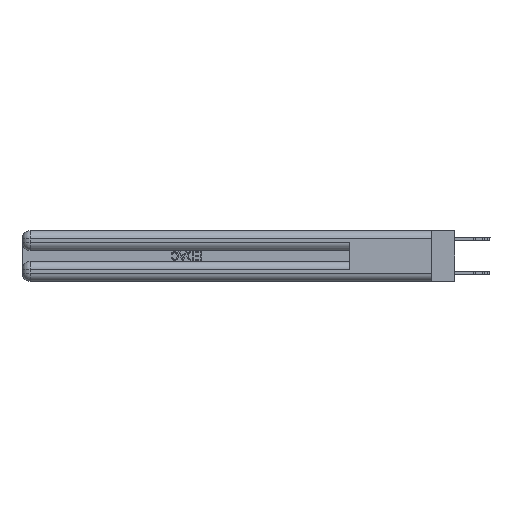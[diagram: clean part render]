
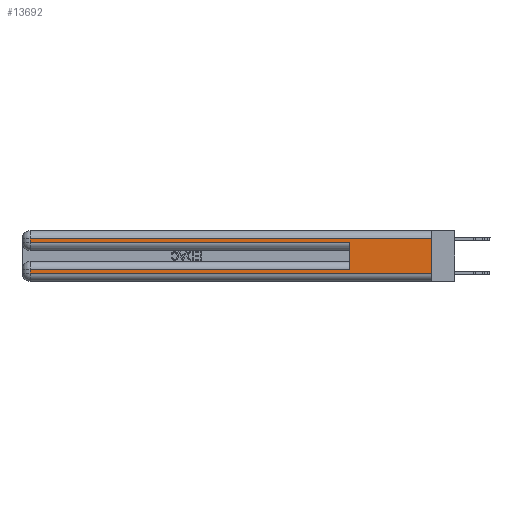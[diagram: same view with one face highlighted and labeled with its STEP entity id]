
A CAD part, left-side view. The second image highlights one B-rep face of the part: STEP entity #13692.
In plain terms, the highlighted planar face has unit normal (-1, 0, 0).
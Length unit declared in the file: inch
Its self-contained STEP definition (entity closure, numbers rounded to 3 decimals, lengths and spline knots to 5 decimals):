
#236 = LINE ( 'NONE', #10302, #12763 ) ;
#909 = EDGE_CURVE ( 'NONE', #18270, #22150, #18606, .T. ) ;
#1221 = CARTESIAN_POINT ( 'NONE',  ( 0., 2.94, 0.37 ) ) ;
#1953 = VECTOR ( 'NONE', #5404, 39.37008 ) ;
#2802 = EDGE_CURVE ( 'NONE', #17576, #24752, #4021, .T. ) ;
#3401 = LINE ( 'NONE', #13656, #1953 ) ;
#4021 = LINE ( 'NONE', #1221, #25824 ) ;
#4067 = VERTEX_POINT ( 'NONE', #9321 ) ;
#4225 = EDGE_CURVE ( 'NONE', #4067, #22150, #236, .T. ) ;
#4426 = CARTESIAN_POINT ( 'NONE',  ( 0., 2.94, 0.085 ) ) ;
#4803 = VECTOR ( 'NONE', #28341, 39.37008 ) ;
#4826 = DIRECTION ( 'NONE',  ( 0., 1., 0. ) ) ;
#5348 = CARTESIAN_POINT ( 'NONE',  ( 0., 0.6, 0.085 ) ) ;
#5404 = DIRECTION ( 'NONE',  ( 0., 0., -1. ) ) ;
#5659 = VECTOR ( 'NONE', #22503, 39.37008 ) ;
#7192 = ORIENTED_EDGE ( 'NONE', *, *, #2802, .T. ) ;
#8212 = CARTESIAN_POINT ( 'NONE',  ( 0., 0., 0.06 ) ) ;
#8763 = VECTOR ( 'NONE', #24407, 39.37008 ) ;
#9306 = DIRECTION ( 'NONE',  ( 1., 0., 0. ) ) ;
#9321 = CARTESIAN_POINT ( 'NONE',  ( 0., 0., 0.31 ) ) ;
#9666 = VERTEX_POINT ( 'NONE', #4426 ) ;
#9867 = CARTESIAN_POINT ( 'NONE',  ( 0., 2.94, 0.31 ) ) ;
#10302 = CARTESIAN_POINT ( 'NONE',  ( 0., 0., 0.37 ) ) ;
#10973 = ORIENTED_EDGE ( 'NONE', *, *, #909, .T. ) ;
#11294 = DIRECTION ( 'NONE',  ( 0., 0., -1. ) ) ;
#11939 = CARTESIAN_POINT ( 'NONE',  ( 0., 0., 0.085 ) ) ;
#12763 = VECTOR ( 'NONE', #25305, 39.37008 ) ;
#12928 = DIRECTION ( 'NONE',  ( 0., 0., 1. ) ) ;
#13603 = DIRECTION ( 'NONE',  ( 0., 0., -1. ) ) ;
#13656 = CARTESIAN_POINT ( 'NONE',  ( 0., 2.94, 0.37 ) ) ;
#13684 = VECTOR ( 'NONE', #12928, 39.37008 ) ;
#13692 = ADVANCED_FACE ( 'NONE', ( #31259 ), #19378, .F. ) ;
#14839 = CARTESIAN_POINT ( 'NONE',  ( 0., 0., 0.285 ) ) ;
#15610 = ORIENTED_EDGE ( 'NONE', *, *, #18496, .T. ) ;
#16903 = LINE ( 'NONE', #24815, #5659 ) ;
#17576 = VERTEX_POINT ( 'NONE', #9867 ) ;
#18212 = VERTEX_POINT ( 'NONE', #5348 ) ;
#18270 = VERTEX_POINT ( 'NONE', #20526 ) ;
#18496 = EDGE_CURVE ( 'NONE', #18212, #9666, #29753, .T. ) ;
#18606 = LINE ( 'NONE', #8212, #4803 ) ;
#19378 = PLANE ( 'NONE',  #30938 ) ;
#20526 = CARTESIAN_POINT ( 'NONE',  ( 0., 2.94, 0.06 ) ) ;
#20727 = EDGE_CURVE ( 'NONE', #24752, #26702, #29842, .T. ) ;
#21183 = CARTESIAN_POINT ( 'NONE',  ( 0., 0., 0.37 ) ) ;
#21469 = CARTESIAN_POINT ( 'NONE',  ( 0., 0.6, 0.285 ) ) ;
#21498 = EDGE_CURVE ( 'NONE', #9666, #18270, #3401, .T. ) ;
#21579 = ORIENTED_EDGE ( 'NONE', *, *, #22158, .T. ) ;
#21739 = CARTESIAN_POINT ( 'NONE',  ( 0., 2.94, 0.285 ) ) ;
#22150 = VERTEX_POINT ( 'NONE', #25139 ) ;
#22158 = EDGE_CURVE ( 'NONE', #4067, #17576, #16903, .T. ) ;
#22503 = DIRECTION ( 'NONE',  ( 0., 1., 0. ) ) ;
#23049 = ORIENTED_EDGE ( 'NONE', *, *, #26531, .F. ) ;
#23849 = ORIENTED_EDGE ( 'NONE', *, *, #20727, .T. ) ;
#24407 = DIRECTION ( 'NONE',  ( 0., -1., 0. ) ) ;
#24712 = EDGE_LOOP ( 'NONE', ( #29784, #21579, #7192, #23849, #23049, #15610, #28738, #10973 ) ) ;
#24752 = VERTEX_POINT ( 'NONE', #21739 ) ;
#24815 = CARTESIAN_POINT ( 'NONE',  ( 0., 0., 0.31 ) ) ;
#25130 = LINE ( 'NONE', #25606, #13684 ) ;
#25139 = CARTESIAN_POINT ( 'NONE',  ( 0., 0., 0.06 ) ) ;
#25305 = DIRECTION ( 'NONE',  ( 0., 0., -1. ) ) ;
#25606 = CARTESIAN_POINT ( 'NONE',  ( 0., 0.6, 0.145 ) ) ;
#25824 = VECTOR ( 'NONE', #11294, 39.37008 ) ;
#26531 = EDGE_CURVE ( 'NONE', #18212, #26702, #25130, .T. ) ;
#26702 = VERTEX_POINT ( 'NONE', #21469 ) ;
#28341 = DIRECTION ( 'NONE',  ( 0., -1., 0. ) ) ;
#28738 = ORIENTED_EDGE ( 'NONE', *, *, #21498, .T. ) ;
#29751 = VECTOR ( 'NONE', #4826, 39.37008 ) ;
#29753 = LINE ( 'NONE', #11939, #29751 ) ;
#29784 = ORIENTED_EDGE ( 'NONE', *, *, #4225, .F. ) ;
#29842 = LINE ( 'NONE', #14839, #8763 ) ;
#30938 = AXIS2_PLACEMENT_3D ( 'NONE', #21183, #9306, #13603 ) ;
#31259 = FACE_OUTER_BOUND ( 'NONE', #24712, .T. ) ;
